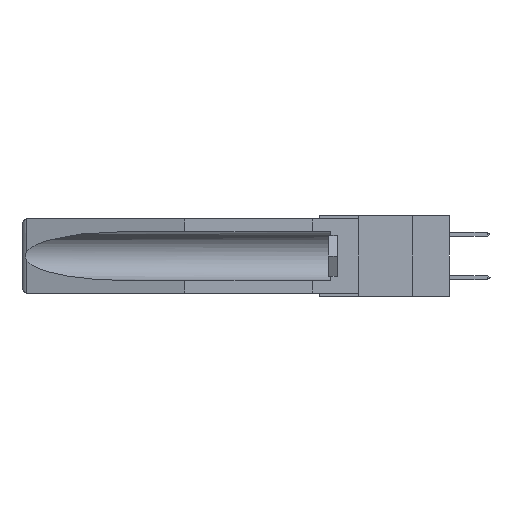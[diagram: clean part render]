
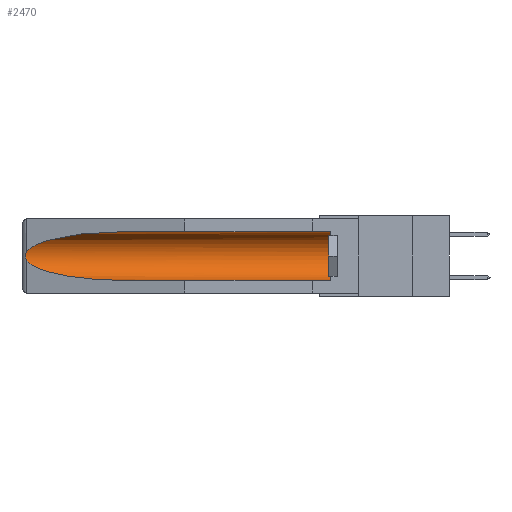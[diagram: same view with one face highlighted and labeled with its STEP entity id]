
A CAD part, left-side view. The second image highlights one B-rep face of the part: STEP entity #2470.
In plain terms, the highlighted cylindrical face has radius 2.857 mm (diameter 5.715 mm), a partial arc.
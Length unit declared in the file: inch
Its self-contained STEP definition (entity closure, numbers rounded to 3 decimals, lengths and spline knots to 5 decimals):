
#460 = ORIENTED_EDGE ( 'NONE', *, *, #1710, .T. ) ;
#849 = VECTOR ( 'NONE', #7532, 39.37008 ) ;
#1330 = CARTESIAN_POINT ( 'NONE',  ( 0.2675, 1.53308, -0.17534 ) ) ;
#1361 = CARTESIAN_POINT ( 'NONE',  ( 0.25451, 1.48313, -0.09465 ) ) ;
#1710 = EDGE_CURVE ( 'NONE', #5107, #19898, #11011, .T. ) ;
#2127 = ORIENTED_EDGE ( 'NONE', *, *, #10361, .T. ) ;
#2260 = EDGE_CURVE ( 'NONE', #18550, #5107, #2682, .T. ) ;
#2441 = DIRECTION ( 'NONE',  ( 0., 0., 1. ) ) ;
#2470 = ADVANCED_FACE ( 'NONE', ( #12549 ), #9721, .F. ) ;
#2682 = CIRCLE ( 'NONE', #8637, 0.1125 ) ;
#2688 =( BOUNDED_CURVE ( )  B_SPLINE_CURVE ( 3, ( #13231, #21426, #6657, #14913 ),
 .UNSPECIFIED., .F., .F. ) 
 B_SPLINE_CURVE_WITH_KNOTS ( ( 4, 4 ),
 ( 0.1948, 1.5708 ),
 .UNSPECIFIED. ) 
 CURVE ( )  GEOMETRIC_REPRESENTATION_ITEM ( )  RATIONAL_B_SPLINE_CURVE ( ( 1., 0.848, 0.848, 1. ) ) 
 REPRESENTATION_ITEM ( '' )  );
#3485 = ORIENTED_EDGE ( 'NONE', *, *, #10324, .F. ) ;
#3872 = CARTESIAN_POINT ( 'NONE',  ( 0.26537, 1.52718, -0.14972 ) ) ;
#4187 = CARTESIAN_POINT ( 'NONE',  ( 0.155, -0.30754, -0.284 ) ) ;
#4460 = DIRECTION ( 'NONE',  ( 0., -1., 0. ) ) ;
#4752 = CARTESIAN_POINT ( 'NONE',  ( 0.26655, 1.53094, -0.18657 ) ) ;
#5107 = VERTEX_POINT ( 'NONE', #17512 ) ;
#5526 = CARTESIAN_POINT ( 'NONE',  ( 0.155, -0.30754, -0.1715 ) ) ;
#6318 = ORIENTED_EDGE ( 'NONE', *, *, #17664, .T. ) ;
#6324 = CARTESIAN_POINT ( 'NONE',  ( 0.155, 1.07973, -0.059 ) ) ;
#6428 = CARTESIAN_POINT ( 'NONE',  ( 0.155, 1.07973, -0.284 ) ) ;
#6657 = CARTESIAN_POINT ( 'NONE',  ( 0.21114, 1.30732, -0.284 ) ) ;
#7169 = EDGE_CURVE ( 'NONE', #16434, #9254, #2688, .T. ) ;
#7460 = CARTESIAN_POINT ( 'NONE',  ( 0.26537, 1.52718, -0.14972 ) ) ;
#7532 = DIRECTION ( 'NONE',  ( 0., 1., 0. ) ) ;
#8464 =( BOUNDED_CURVE ( )  B_SPLINE_CURVE ( 3, ( #6324, #14727, #1361, #19623 ),
 .UNSPECIFIED., .F., .F. ) 
 B_SPLINE_CURVE_WITH_KNOTS ( ( 4, 4 ),
 ( 4.71239, 6.08839 ),
 .UNSPECIFIED. ) 
 CURVE ( )  GEOMETRIC_REPRESENTATION_ITEM ( )  RATIONAL_B_SPLINE_CURVE ( ( 1., 0.848, 0.848, 1. ) ) 
 REPRESENTATION_ITEM ( '' )  );
#8637 = AXIS2_PLACEMENT_3D ( 'NONE', #14391, #4460, #11428 ) ;
#9254 = VERTEX_POINT ( 'NONE', #6428 ) ;
#9651 = CARTESIAN_POINT ( 'NONE',  ( 0.155, -0.30754, -0.059 ) ) ;
#9721 = CYLINDRICAL_SURFACE ( 'NONE', #15298, 0.1125 ) ;
#10324 = EDGE_CURVE ( 'NONE', #18550, #9254, #18090, .T. ) ;
#10361 = EDGE_CURVE ( 'NONE', #15079, #16434, #14278, .T. ) ;
#10562 = DIRECTION ( 'NONE',  ( 0., 1., 0. ) ) ;
#11011 = LINE ( 'NONE', #9651, #18801 ) ;
#11293 = CARTESIAN_POINT ( 'NONE',  ( 0.26597, 1.52961, -0.15275 ) ) ;
#11358 = CARTESIAN_POINT ( 'NONE',  ( 0.2675, 1.53308, -0.16763 ) ) ;
#11428 = DIRECTION ( 'NONE',  ( 0., 0., 1. ) ) ;
#11749 = CARTESIAN_POINT ( 'NONE',  ( 0.26537, 1.52718, -0.19328 ) ) ;
#12549 = FACE_OUTER_BOUND ( 'NONE', #12848, .T. ) ;
#12801 = CARTESIAN_POINT ( 'NONE',  ( 0.26654, 1.53092, -0.15636 ) ) ;
#12848 = EDGE_LOOP ( 'NONE', ( #6318, #2127, #21474, #3485, #13902, #460 ) ) ;
#13007 = CARTESIAN_POINT ( 'NONE',  ( 0.2673, 1.53269, -0.17917 ) ) ;
#13231 = CARTESIAN_POINT ( 'NONE',  ( 0.26537, 1.52718, -0.19328 ) ) ;
#13902 = ORIENTED_EDGE ( 'NONE', *, *, #2260, .T. ) ;
#14278 = B_SPLINE_CURVE_WITH_KNOTS ( 'NONE', 3,
 ( #7460, #11293, #12801, #19662, #11358, #1330, #13007, #4752, #17379, #19085 ),
 .UNSPECIFIED., .F., .F.,
 ( 4, 2, 2, 2, 4 ),
 ( 0., 0.00029, 0.00058, 0.00087, 0.00117 ),
 .UNSPECIFIED. ) ;
#14391 = CARTESIAN_POINT ( 'NONE',  ( 0.155, 0.126, -0.1715 ) ) ;
#14727 = CARTESIAN_POINT ( 'NONE',  ( 0.21114, 1.30732, -0.059 ) ) ;
#14904 = CARTESIAN_POINT ( 'NONE',  ( 0.155, 0.126, -0.284 ) ) ;
#14913 = CARTESIAN_POINT ( 'NONE',  ( 0.155, 1.07973, -0.284 ) ) ;
#15079 = VERTEX_POINT ( 'NONE', #3872 ) ;
#15298 = AXIS2_PLACEMENT_3D ( 'NONE', #5526, #10562, #2441 ) ;
#16301 = DIRECTION ( 'NONE',  ( 0., 1., 0. ) ) ;
#16434 = VERTEX_POINT ( 'NONE', #11749 ) ;
#17379 = CARTESIAN_POINT ( 'NONE',  ( 0.26597, 1.5296, -0.19026 ) ) ;
#17512 = CARTESIAN_POINT ( 'NONE',  ( 0.155, 0.126, -0.059 ) ) ;
#17664 = EDGE_CURVE ( 'NONE', #19898, #15079, #8464, .T. ) ;
#18090 = LINE ( 'NONE', #4187, #849 ) ;
#18550 = VERTEX_POINT ( 'NONE', #14904 ) ;
#18625 = CARTESIAN_POINT ( 'NONE',  ( 0.155, 1.07973, -0.059 ) ) ;
#18801 = VECTOR ( 'NONE', #16301, 39.37008 ) ;
#19085 = CARTESIAN_POINT ( 'NONE',  ( 0.26537, 1.52718, -0.19328 ) ) ;
#19623 = CARTESIAN_POINT ( 'NONE',  ( 0.26537, 1.52718, -0.14972 ) ) ;
#19662 = CARTESIAN_POINT ( 'NONE',  ( 0.2673, 1.5327, -0.16383 ) ) ;
#19898 = VERTEX_POINT ( 'NONE', #18625 ) ;
#21426 = CARTESIAN_POINT ( 'NONE',  ( 0.25451, 1.48313, -0.24835 ) ) ;
#21474 = ORIENTED_EDGE ( 'NONE', *, *, #7169, .T. ) ;
